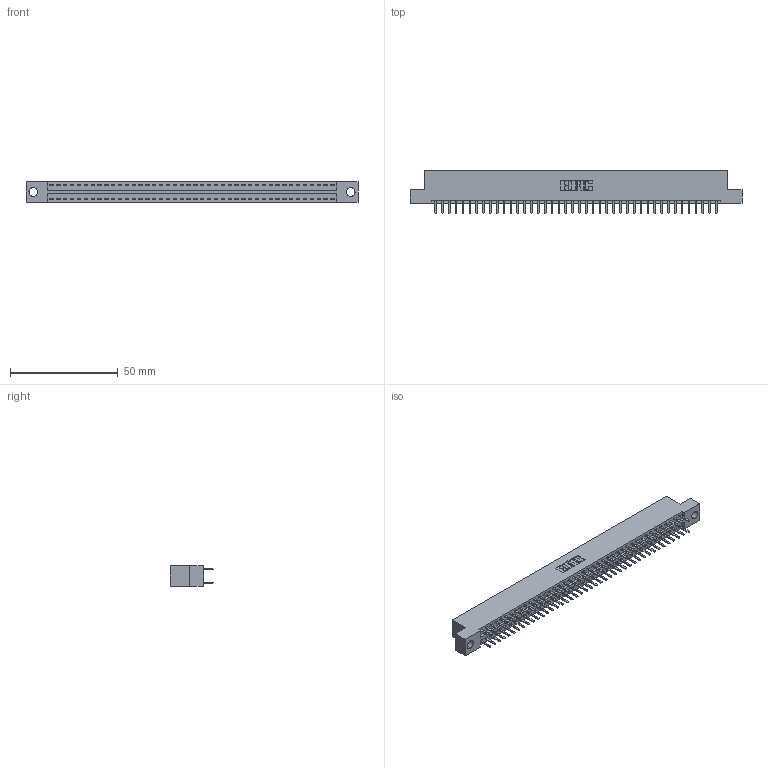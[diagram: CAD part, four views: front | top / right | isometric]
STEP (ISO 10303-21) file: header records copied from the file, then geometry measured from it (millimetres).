
FILE_DESCRIPTION (( 'STEP AP203' ), '1' );
FILE_NAME ('396-084-520-204.STEP', '2019-10-30T23:47:36', ( '' ), ( '' ), 'SwSTEP 2.0', 'SolidWorks 2016', '' );
FILE_SCHEMA (( 'CONFIG_CONTROL_DESIGN' ));
Length unit declared in the file: inch
Products named in the file (3): 346 Part_Flush Mounting Lugs - 0.156 Dia-TH; 396-084-520-204; 345-292-001_345-293-120
Assembly tree (85 placements, depth 2):
  396-084-520-204
    346 Part_Flush Mounting Lugs - 0.156 Dia-TH
    345-292-001_345-293-120  x84
Bounding box: 153.92 x 20.02 x 9.4 mm (x, y, z)
Volume: 14884.7 mm3; surface area: 20186.9 mm2
Topology: 85 solids, 85 shells, 4826 faces, 14021 edges, 9122 vertices
Faces by surface type: plane 3184, cylinder 1642
Entity records: 27527 total; most frequent: CARTESIAN_POINT 4548, ORIENTED_EDGE 4470, DIRECTION 4047, EDGE_CURVE 2235, VECTOR 1931, LINE 1931, VERTEX_POINT 1486, AXIS2_PLACEMENT_3D 1058
